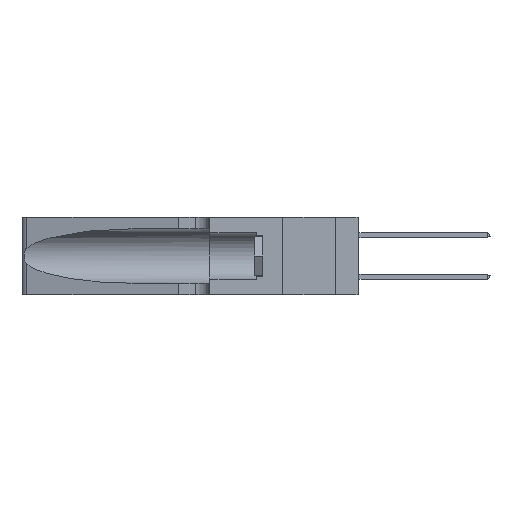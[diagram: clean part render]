
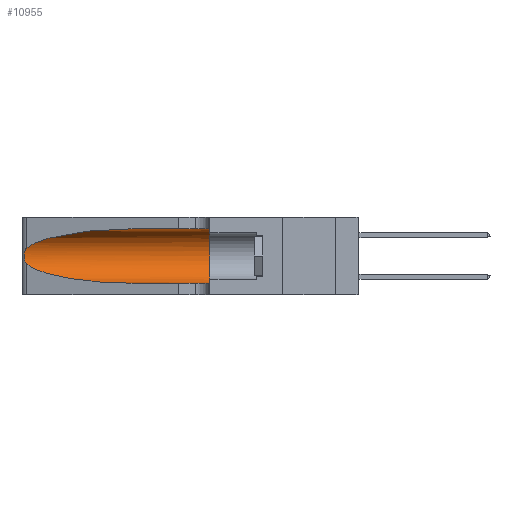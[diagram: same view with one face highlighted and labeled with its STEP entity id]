
A CAD part, left-side view. The second image highlights one B-rep face of the part: STEP entity #10955.
In plain terms, the highlighted cylindrical face has radius 3.308 mm (diameter 6.617 mm), a partial arc.
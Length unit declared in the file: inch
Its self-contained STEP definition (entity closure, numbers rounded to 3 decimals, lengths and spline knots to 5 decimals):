
#361 = LINE ( 'NONE', #19530, #21929 ) ;
#804 = CARTESIAN_POINT ( 'NONE',  ( 0.1305, 1.61858, 0.05475 ) ) ;
#1929 = CARTESIAN_POINT ( 'NONE',  ( 0.1305, 0.72297, 0.31525 ) ) ;
#1978 = CARTESIAN_POINT ( 'NONE',  ( 0.25789, 1.23486, 0.15765 ) ) ;
#2232 = EDGE_CURVE ( 'NONE', #25216, #8175, #7635, .T. ) ;
#3028 = VERTEX_POINT ( 'NONE', #20470 ) ;
#4007 = CARTESIAN_POINT ( 'NONE',  ( 0.25487, 1.22718, 0.22369 ) ) ;
#4096 = CARTESIAN_POINT ( 'NONE',  ( 0.25555, 1.22993, 0.14849 ) ) ;
#4112 = CYLINDRICAL_SURFACE ( 'NONE', #13604, 0.13025 ) ;
#4611 = ORIENTED_EDGE ( 'NONE', *, *, #10628, .F. ) ;
#4978 = VERTEX_POINT ( 'NONE', #5739 ) ;
#5651 =( BOUNDED_CURVE ( )  B_SPLINE_CURVE ( 3, ( #1929, #14126, #18136, #6109 ),
 .UNSPECIFIED., .F., .T. ) 
 B_SPLINE_CURVE_WITH_KNOTS ( ( 4, 4 ),
 ( 1.5708, 2.84003 ),
 .UNSPECIFIED. ) 
 CURVE ( )  GEOMETRIC_REPRESENTATION_ITEM ( )  RATIONAL_B_SPLINE_CURVE ( ( 1., 0.87, 0.87, 1. ) ) 
 REPRESENTATION_ITEM ( '' )  );
#5739 = CARTESIAN_POINT ( 'NONE',  ( 0.25487, 1.22718, 0.22369 ) ) ;
#6109 = CARTESIAN_POINT ( 'NONE',  ( 0.25487, 1.22718, 0.22369 ) ) ;
#6524 = LINE ( 'NONE', #804, #21851 ) ;
#7634 = CARTESIAN_POINT ( 'NONE',  ( 0.25487, 1.22718, 0.14631 ) ) ;
#7635 =( BOUNDED_CURVE ( )  B_SPLINE_CURVE ( 3, ( #10246, #8211, #22156, #24144 ),
 .UNSPECIFIED., .F., .T. ) 
 B_SPLINE_CURVE_WITH_KNOTS ( ( 4, 4 ),
 ( 3.44316, 4.71239 ),
 .UNSPECIFIED. ) 
 CURVE ( )  GEOMETRIC_REPRESENTATION_ITEM ( )  RATIONAL_B_SPLINE_CURVE ( ( 1., 0.87, 0.87, 1. ) ) 
 REPRESENTATION_ITEM ( '' )  );
#8139 = ORIENTED_EDGE ( 'NONE', *, *, #2232, .T. ) ;
#8151 = CARTESIAN_POINT ( 'NONE',  ( 0.25787, 1.23484, 0.2124 ) ) ;
#8175 = VERTEX_POINT ( 'NONE', #13243 ) ;
#8211 = CARTESIAN_POINT ( 'NONE',  ( 0.2373, 1.15595, 0.08982 ) ) ;
#9606 = DIRECTION ( 'NONE',  ( 0., -1., 0. ) ) ;
#10115 = AXIS2_PLACEMENT_3D ( 'NONE', #10511, #24409, #12506 ) ;
#10178 = CARTESIAN_POINT ( 'NONE',  ( 0.26018, 1.23835, 0.19895 ) ) ;
#10246 = CARTESIAN_POINT ( 'NONE',  ( 0.25487, 1.22718, 0.14631 ) ) ;
#10511 = CARTESIAN_POINT ( 'NONE',  ( 0.1305, 0.35, 0.185 ) ) ;
#10628 = EDGE_CURVE ( 'NONE', #3028, #19379, #17688, .T. ) ;
#10955 = ADVANCED_FACE ( 'NONE', ( #14856 ), #4112, .F. ) ;
#11431 = DIRECTION ( 'NONE',  ( 0., 0., -1. ) ) ;
#12157 = CARTESIAN_POINT ( 'NONE',  ( 0.26075, 1.23896, 0.178 ) ) ;
#12506 = DIRECTION ( 'NONE',  ( 0., 0., 1. ) ) ;
#13063 = DIRECTION ( 'NONE',  ( 0., -1., 0. ) ) ;
#13099 = ORIENTED_EDGE ( 'NONE', *, *, #24423, .T. ) ;
#13243 = CARTESIAN_POINT ( 'NONE',  ( 0.1305, 0.72297, 0.05475 ) ) ;
#13604 = AXIS2_PLACEMENT_3D ( 'NONE', #23373, #21352, #11431 ) ;
#13815 = EDGE_CURVE ( 'NONE', #8175, #19379, #6524, .T. ) ;
#14126 = CARTESIAN_POINT ( 'NONE',  ( 0.18966, 0.96281, 0.31525 ) ) ;
#14180 = CARTESIAN_POINT ( 'NONE',  ( 0.25856, 1.23593, 0.16098 ) ) ;
#14856 = FACE_OUTER_BOUND ( 'NONE', #25357, .T. ) ;
#16182 = CARTESIAN_POINT ( 'NONE',  ( 0.25639, 1.23186, 0.15144 ) ) ;
#17688 = CIRCLE ( 'NONE', #10115, 0.13025 ) ;
#17717 = B_SPLINE_CURVE_WITH_KNOTS ( 'NONE', 3,
 ( #4007, #24000, #20089, #8151, #22091, #10178, #24082, #12157, #26084, #14180, #1978, #16182, #4096, #18183 ),
 .UNSPECIFIED., .F., .F.,
 ( 4, 2, 2, 2, 2, 2, 4 ),
 ( 0., 0.00027, 0.00053, 0.00107, 0.0016, 0.00187, 0.00214 ),
 .UNSPECIFIED. ) ;
#17805 = ORIENTED_EDGE ( 'NONE', *, *, #13815, .T. ) ;
#18136 = CARTESIAN_POINT ( 'NONE',  ( 0.2373, 1.15595, 0.28018 ) ) ;
#18183 = CARTESIAN_POINT ( 'NONE',  ( 0.25487, 1.22718, 0.14631 ) ) ;
#19379 = VERTEX_POINT ( 'NONE', #22788 ) ;
#19530 = CARTESIAN_POINT ( 'NONE',  ( 0.1305, 1.61858, 0.31525 ) ) ;
#20089 = CARTESIAN_POINT ( 'NONE',  ( 0.25639, 1.23184, 0.21858 ) ) ;
#20183 = EDGE_CURVE ( 'NONE', #24668, #3028, #361, .T. ) ;
#20355 = EDGE_CURVE ( 'NONE', #24668, #4978, #5651, .T. ) ;
#20470 = CARTESIAN_POINT ( 'NONE',  ( 0.1305, 0.35, 0.31525 ) ) ;
#21352 = DIRECTION ( 'NONE',  ( 0., -1., 0. ) ) ;
#21851 = VECTOR ( 'NONE', #13063, 39.37008 ) ;
#21929 = VECTOR ( 'NONE', #9606, 39.37008 ) ;
#22091 = CARTESIAN_POINT ( 'NONE',  ( 0.25854, 1.2359, 0.20912 ) ) ;
#22156 = CARTESIAN_POINT ( 'NONE',  ( 0.18966, 0.96281, 0.05475 ) ) ;
#22407 = ORIENTED_EDGE ( 'NONE', *, *, #20183, .F. ) ;
#22788 = CARTESIAN_POINT ( 'NONE',  ( 0.1305, 0.35, 0.05475 ) ) ;
#22872 = CARTESIAN_POINT ( 'NONE',  ( 0.1305, 0.72297, 0.31525 ) ) ;
#23373 = CARTESIAN_POINT ( 'NONE',  ( 0.1305, 1.61858, 0.185 ) ) ;
#24000 = CARTESIAN_POINT ( 'NONE',  ( 0.25555, 1.22994, 0.2215 ) ) ;
#24082 = CARTESIAN_POINT ( 'NONE',  ( 0.26075, 1.23896, 0.19203 ) ) ;
#24144 = CARTESIAN_POINT ( 'NONE',  ( 0.1305, 0.72297, 0.05475 ) ) ;
#24409 = DIRECTION ( 'NONE',  ( 0., 1., 0. ) ) ;
#24423 = EDGE_CURVE ( 'NONE', #4978, #25216, #17717, .T. ) ;
#24668 = VERTEX_POINT ( 'NONE', #22872 ) ;
#25003 = ORIENTED_EDGE ( 'NONE', *, *, #20355, .T. ) ;
#25216 = VERTEX_POINT ( 'NONE', #7634 ) ;
#25357 = EDGE_LOOP ( 'NONE', ( #25003, #13099, #8139, #17805, #4611, #22407 ) ) ;
#26084 = CARTESIAN_POINT ( 'NONE',  ( 0.26017, 1.23833, 0.17102 ) ) ;
